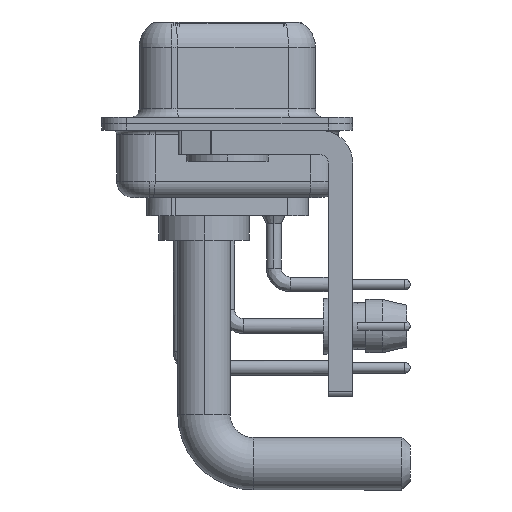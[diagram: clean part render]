
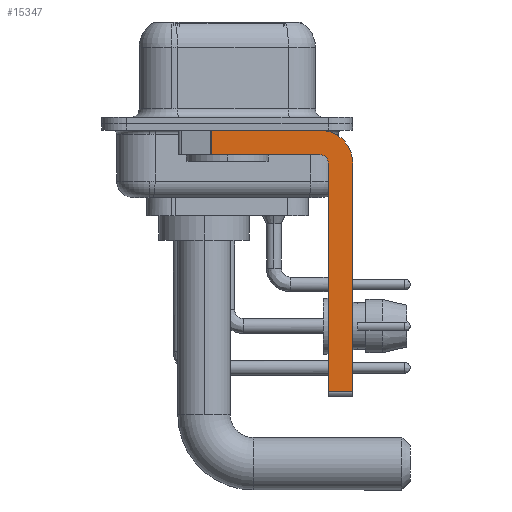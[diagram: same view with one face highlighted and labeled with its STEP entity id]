
A CAD part, left-side view. The second image highlights one B-rep face of the part: STEP entity #15347.
In plain terms, the highlighted planar face has unit normal (-1, 0, 0).
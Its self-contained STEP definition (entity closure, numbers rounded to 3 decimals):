
#429 = VERTEX_POINT ( 'NONE', #26715 ) ;
#911 = LINE ( 'NONE', #17932, #26438 ) ;
#1654 = VERTEX_POINT ( 'NONE', #13445 ) ;
#2208 = DIRECTION ( 'NONE',  ( 0., 1., 0. ) ) ;
#2485 = VERTEX_POINT ( 'NONE', #26729 ) ;
#2585 = ORIENTED_EDGE ( 'NONE', *, *, #30391, .F. ) ;
#3238 = CARTESIAN_POINT ( 'NONE',  ( -2.9, -6.15, -16.35 ) ) ;
#3636 = DIRECTION ( 'NONE',  ( 0., 0., 1. ) ) ;
#4319 = EDGE_CURVE ( 'NONE', #2485, #11965, #6522, .T. ) ;
#5542 = CARTESIAN_POINT ( 'NONE',  ( -2.9, -5.65, -2.4 ) ) ;
#5701 = DIRECTION ( 'NONE',  ( 1., 0., 0. ) ) ;
#6127 = DIRECTION ( 'NONE',  ( 1., 0., 0. ) ) ;
#6508 = AXIS2_PLACEMENT_3D ( 'NONE', #25775, #10990, #27867 ) ;
#6522 = LINE ( 'NONE', #26261, #15766 ) ;
#6719 = CARTESIAN_POINT ( 'NONE',  ( -2.9, 3., -0.4 ) ) ;
#6838 = CARTESIAN_POINT ( 'NONE',  ( -2.9, 0.978, -0.4 ) ) ;
#7147 = EDGE_CURVE ( 'NONE', #7511, #429, #11984, .T. ) ;
#7511 = VERTEX_POINT ( 'NONE', #30745 ) ;
#8678 = CARTESIAN_POINT ( 'NONE',  ( -2.9, -5.65, -2.4 ) ) ;
#8963 = LINE ( 'NONE', #6719, #9739 ) ;
#9032 = LINE ( 'NONE', #18837, #16226 ) ;
#9739 = VECTOR ( 'NONE', #29025, 1000. ) ;
#10491 = EDGE_LOOP ( 'NONE', ( #20892, #26277, #12705, #31682, #17928, #17048, #31337, #2585 ) ) ;
#10990 = DIRECTION ( 'NONE',  ( -1., 0., 0. ) ) ;
#11307 = DIRECTION ( 'NONE',  ( 0., 0., -1. ) ) ;
#11795 = VERTEX_POINT ( 'NONE', #6838 ) ;
#11965 = VERTEX_POINT ( 'NONE', #12559 ) ;
#11984 = LINE ( 'NONE', #14403, #28161 ) ;
#12559 = CARTESIAN_POINT ( 'NONE',  ( -2.9, -7.65, -16.35 ) ) ;
#12705 = ORIENTED_EDGE ( 'NONE', *, *, #7147, .F. ) ;
#13104 = VECTOR ( 'NONE', #3636, 1000. ) ;
#13445 = CARTESIAN_POINT ( 'NONE',  ( -2.9, -6.15, -2.4 ) ) ;
#13803 = PLANE ( 'NONE',  #28058 ) ;
#13997 = DIRECTION ( 'NONE',  ( 0., -1., 0. ) ) ;
#14403 = CARTESIAN_POINT ( 'NONE',  ( -2.9, -5.65, -1.9 ) ) ;
#14873 = EDGE_CURVE ( 'NONE', #1654, #7511, #24438, .T. ) ;
#15246 = VERTEX_POINT ( 'NONE', #3238 ) ;
#15347 = ADVANCED_FACE ( 'NONE', ( #16213 ), #13803, .F. ) ;
#15766 = VECTOR ( 'NONE', #11307, 1000. ) ;
#15814 = LINE ( 'NONE', #25615, #13104 ) ;
#16051 = DIRECTION ( 'NONE',  ( 0., 0., -1. ) ) ;
#16213 = FACE_OUTER_BOUND ( 'NONE', #10491, .T. ) ;
#16226 = VECTOR ( 'NONE', #13997, 1000. ) ;
#16618 = CIRCLE ( 'NONE', #18196, 2. ) ;
#17048 = ORIENTED_EDGE ( 'NONE', *, *, #25668, .T. ) ;
#17212 = EDGE_CURVE ( 'NONE', #11795, #23442, #8963, .T. ) ;
#17928 = ORIENTED_EDGE ( 'NONE', *, *, #25062, .F. ) ;
#17932 = CARTESIAN_POINT ( 'NONE',  ( -2.9, 0.978, -1.9 ) ) ;
#18196 = AXIS2_PLACEMENT_3D ( 'NONE', #5542, #5701, #25269 ) ;
#18837 = CARTESIAN_POINT ( 'NONE',  ( -2.9, -5.65, -16.35 ) ) ;
#20674 = DIRECTION ( 'NONE',  ( 0., 0., -1. ) ) ;
#20892 = ORIENTED_EDGE ( 'NONE', *, *, #17212, .F. ) ;
#23442 = VERTEX_POINT ( 'NONE', #31271 ) ;
#24438 = CIRCLE ( 'NONE', #6508, 0.5 ) ;
#24535 = EDGE_CURVE ( 'NONE', #11795, #429, #911, .T. ) ;
#25062 = EDGE_CURVE ( 'NONE', #15246, #1654, #15814, .T. ) ;
#25269 = DIRECTION ( 'NONE',  ( 0., 0., -1. ) ) ;
#25615 = CARTESIAN_POINT ( 'NONE',  ( -2.9, -6.15, -16.6 ) ) ;
#25668 = EDGE_CURVE ( 'NONE', #15246, #11965, #9032, .T. ) ;
#25775 = CARTESIAN_POINT ( 'NONE',  ( -2.9, -5.65, -2.4 ) ) ;
#26261 = CARTESIAN_POINT ( 'NONE',  ( -2.9, -7.65, -2.4 ) ) ;
#26277 = ORIENTED_EDGE ( 'NONE', *, *, #24535, .T. ) ;
#26438 = VECTOR ( 'NONE', #20674, 1000. ) ;
#26715 = CARTESIAN_POINT ( 'NONE',  ( -2.9, 0.978, -1.9 ) ) ;
#26729 = CARTESIAN_POINT ( 'NONE',  ( -2.9, -7.65, -2.4 ) ) ;
#27867 = DIRECTION ( 'NONE',  ( 0., 0., 1. ) ) ;
#28058 = AXIS2_PLACEMENT_3D ( 'NONE', #8678, #6127, #16051 ) ;
#28161 = VECTOR ( 'NONE', #2208, 1000. ) ;
#29025 = DIRECTION ( 'NONE',  ( 0., -1., 0. ) ) ;
#30391 = EDGE_CURVE ( 'NONE', #23442, #2485, #16618, .T. ) ;
#30745 = CARTESIAN_POINT ( 'NONE',  ( -2.9, -5.65, -1.9 ) ) ;
#31271 = CARTESIAN_POINT ( 'NONE',  ( -2.9, -5.65, -0.4 ) ) ;
#31337 = ORIENTED_EDGE ( 'NONE', *, *, #4319, .F. ) ;
#31682 = ORIENTED_EDGE ( 'NONE', *, *, #14873, .F. ) ;
